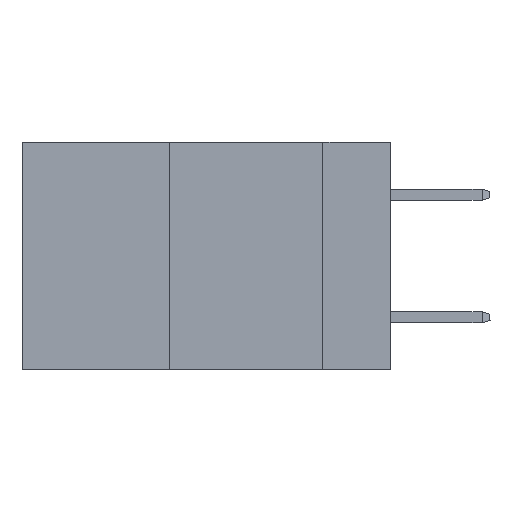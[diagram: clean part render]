
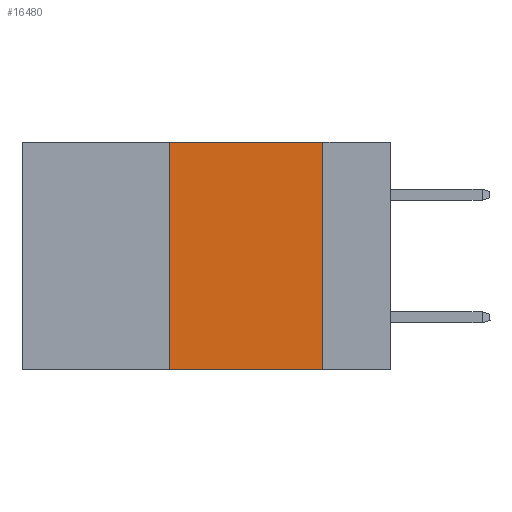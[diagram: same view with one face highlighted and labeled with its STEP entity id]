
A CAD part, left-side view. The second image highlights one B-rep face of the part: STEP entity #16480.
In plain terms, the highlighted planar face has unit normal (-1, 0, 0).
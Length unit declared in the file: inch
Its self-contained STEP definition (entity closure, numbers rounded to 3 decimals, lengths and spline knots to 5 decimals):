
#199 = LINE ( 'NONE', #11937, #1939 ) ;
#666 = VERTEX_POINT ( 'NONE', #15120 ) ;
#1364 = ORIENTED_EDGE ( 'NONE', *, *, #2371, .F. ) ;
#1939 = VECTOR ( 'NONE', #13853, 39.37008 ) ;
#2371 = EDGE_CURVE ( 'NONE', #8634, #8669, #199, .T. ) ;
#3552 = FACE_OUTER_BOUND ( 'NONE', #3792, .T. ) ;
#3792 = EDGE_LOOP ( 'NONE', ( #1364, #8889, #15188, #21526 ) ) ;
#4513 = CARTESIAN_POINT ( 'NONE',  ( 0., 0.6, 0. ) ) ;
#4928 = VECTOR ( 'NONE', #21240, 39.37008 ) ;
#4934 = AXIS2_PLACEMENT_3D ( 'NONE', #19839, #18567, #22351 ) ;
#5372 = EDGE_CURVE ( 'NONE', #666, #8634, #13329, .T. ) ;
#5910 = LINE ( 'NONE', #20865, #12258 ) ;
#8634 = VERTEX_POINT ( 'NONE', #21935 ) ;
#8669 = VERTEX_POINT ( 'NONE', #23703 ) ;
#8889 = ORIENTED_EDGE ( 'NONE', *, *, #5372, .F. ) ;
#10025 = CARTESIAN_POINT ( 'NONE',  ( 0., 0.36, -0.37 ) ) ;
#11553 = VECTOR ( 'NONE', #19507, 39.37008 ) ;
#11937 = CARTESIAN_POINT ( 'NONE',  ( 0., 0.11, 0. ) ) ;
#12258 = VECTOR ( 'NONE', #17332, 39.37008 ) ;
#13329 = LINE ( 'NONE', #4513, #4928 ) ;
#13853 = DIRECTION ( 'NONE',  ( 0., 0., -1. ) ) ;
#15120 = CARTESIAN_POINT ( 'NONE',  ( 0., 0.36, 0. ) ) ;
#15188 = ORIENTED_EDGE ( 'NONE', *, *, #17750, .F. ) ;
#15813 = CARTESIAN_POINT ( 'NONE',  ( 0., 0.36, 0. ) ) ;
#16480 = ADVANCED_FACE ( 'NONE', ( #3552 ), #18013, .F. ) ;
#17332 = DIRECTION ( 'NONE',  ( 0., -1., 0. ) ) ;
#17512 = VERTEX_POINT ( 'NONE', #10025 ) ;
#17750 = EDGE_CURVE ( 'NONE', #17512, #666, #17966, .T. ) ;
#17966 = LINE ( 'NONE', #15813, #11553 ) ;
#18013 = PLANE ( 'NONE',  #4934 ) ;
#18567 = DIRECTION ( 'NONE',  ( 1., 0., 0. ) ) ;
#19507 = DIRECTION ( 'NONE',  ( 0., 0., 1. ) ) ;
#19839 = CARTESIAN_POINT ( 'NONE',  ( 0., 0.6, 0. ) ) ;
#20477 = EDGE_CURVE ( 'NONE', #17512, #8669, #5910, .T. ) ;
#20865 = CARTESIAN_POINT ( 'NONE',  ( 0., 0.6, -0.37 ) ) ;
#21240 = DIRECTION ( 'NONE',  ( 0., -1., 0. ) ) ;
#21526 = ORIENTED_EDGE ( 'NONE', *, *, #20477, .T. ) ;
#21935 = CARTESIAN_POINT ( 'NONE',  ( 0., 0.11, 0. ) ) ;
#22351 = DIRECTION ( 'NONE',  ( 0., 0., -1. ) ) ;
#23703 = CARTESIAN_POINT ( 'NONE',  ( 0., 0.11, -0.37 ) ) ;
